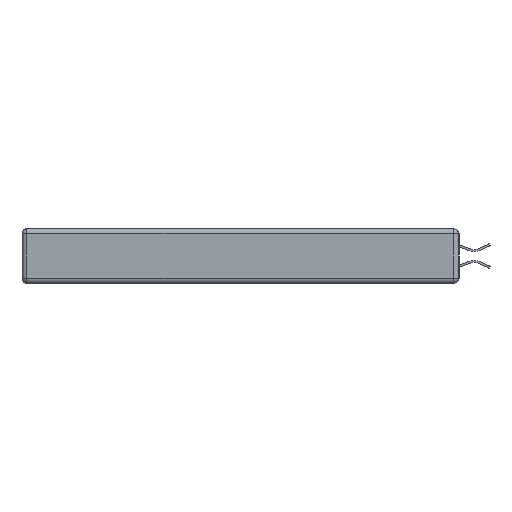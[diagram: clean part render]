
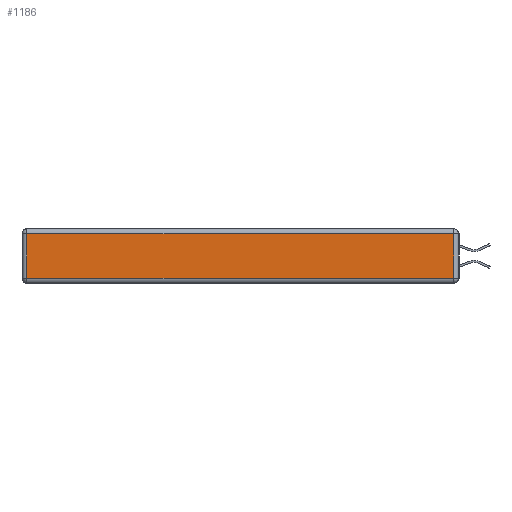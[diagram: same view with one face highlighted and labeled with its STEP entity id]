
A CAD part, left-side view. The second image highlights one B-rep face of the part: STEP entity #1186.
In plain terms, the highlighted planar face has unit normal (-1, 0, 0).
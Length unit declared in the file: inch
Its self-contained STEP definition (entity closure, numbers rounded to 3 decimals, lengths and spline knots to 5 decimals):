
#1186 = ADVANCED_FACE ( 'NONE', ( #4196 ), #1624, .T. ) ;
#1464 = VECTOR ( 'NONE', #8325, 39.37008 ) ;
#1624 = PLANE ( 'NONE',  #14417 ) ;
#3988 = CARTESIAN_POINT ( 'NONE',  ( 0., 2.72, -0.313 ) ) ;
#4196 = FACE_OUTER_BOUND ( 'NONE', #8848, .T. ) ;
#4822 = DIRECTION ( 'NONE',  ( 0., 0., -1. ) ) ;
#6623 = DIRECTION ( 'NONE',  ( 0., 0., 1. ) ) ;
#7260 = EDGE_CURVE ( 'NONE', #11150, #27905, #31214, .T. ) ;
#7911 = ORIENTED_EDGE ( 'NONE', *, *, #19826, .T. ) ;
#8325 = DIRECTION ( 'NONE',  ( 0., 0., 1. ) ) ;
#8848 = EDGE_LOOP ( 'NONE', ( #28249, #32896, #7911, #28662 ) ) ;
#9012 = CARTESIAN_POINT ( 'NONE',  ( 0., 0.03, -0.313 ) ) ;
#11150 = VERTEX_POINT ( 'NONE', #3988 ) ;
#14417 = AXIS2_PLACEMENT_3D ( 'NONE', #25083, #27595, #6623 ) ;
#15015 = LINE ( 'NONE', #24102, #1464 ) ;
#15490 = LINE ( 'NONE', #25739, #15919 ) ;
#15630 = DIRECTION ( 'NONE',  ( 0., -1., 0. ) ) ;
#15634 = CARTESIAN_POINT ( 'NONE',  ( 0., 0.03, -0.03 ) ) ;
#15919 = VECTOR ( 'NONE', #4822, 39.37008 ) ;
#19826 = EDGE_CURVE ( 'NONE', #28239, #28531, #23261, .T. ) ;
#23261 = LINE ( 'NONE', #25910, #25286 ) ;
#24102 = CARTESIAN_POINT ( 'NONE',  ( 0., 0.03, -0.343 ) ) ;
#25083 = CARTESIAN_POINT ( 'NONE',  ( 0., 0., -0.343 ) ) ;
#25286 = VECTOR ( 'NONE', #31408, 39.37008 ) ;
#25739 = CARTESIAN_POINT ( 'NONE',  ( 0., 2.72, -0.343 ) ) ;
#25910 = CARTESIAN_POINT ( 'NONE',  ( 0., 2.75, -0.03 ) ) ;
#26059 = EDGE_CURVE ( 'NONE', #28531, #11150, #15490, .T. ) ;
#27595 = DIRECTION ( 'NONE',  ( -1., 0., 0. ) ) ;
#27905 = VERTEX_POINT ( 'NONE', #9012 ) ;
#28239 = VERTEX_POINT ( 'NONE', #15634 ) ;
#28249 = ORIENTED_EDGE ( 'NONE', *, *, #7260, .T. ) ;
#28507 = CARTESIAN_POINT ( 'NONE',  ( 0., 0., -0.313 ) ) ;
#28531 = VERTEX_POINT ( 'NONE', #28579 ) ;
#28579 = CARTESIAN_POINT ( 'NONE',  ( 0., 2.72, -0.03 ) ) ;
#28662 = ORIENTED_EDGE ( 'NONE', *, *, #26059, .T. ) ;
#29576 = VECTOR ( 'NONE', #15630, 39.37008 ) ;
#31214 = LINE ( 'NONE', #28507, #29576 ) ;
#31408 = DIRECTION ( 'NONE',  ( 0., 1., 0. ) ) ;
#31618 = EDGE_CURVE ( 'NONE', #27905, #28239, #15015, .T. ) ;
#32896 = ORIENTED_EDGE ( 'NONE', *, *, #31618, .T. ) ;
